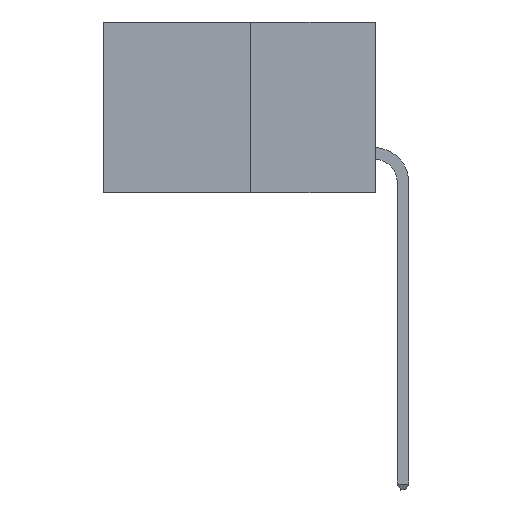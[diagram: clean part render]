
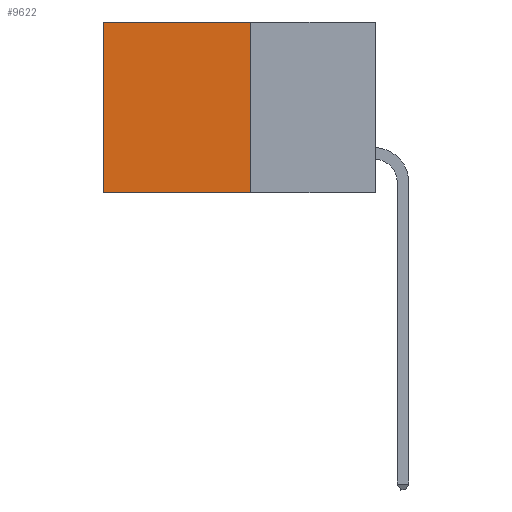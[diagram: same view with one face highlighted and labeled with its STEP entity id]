
A CAD part, left-side view. The second image highlights one B-rep face of the part: STEP entity #9622.
In plain terms, the highlighted planar face has unit normal (-1, 0, 0).
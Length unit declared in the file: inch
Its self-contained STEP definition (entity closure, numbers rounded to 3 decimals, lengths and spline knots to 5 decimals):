
#158 = DIRECTION ( 'NONE',  ( 0., 0., -1. ) ) ;
#978 = VERTEX_POINT ( 'NONE', #2963 ) ;
#1061 = CARTESIAN_POINT ( 'NONE',  ( 0.277, 0.27, -0.37 ) ) ;
#1401 = DIRECTION ( 'NONE',  ( 0., 1., 0. ) ) ;
#1878 = LINE ( 'NONE', #3910, #11128 ) ;
#1903 = CARTESIAN_POINT ( 'NONE',  ( 0.277, 0.59, 0. ) ) ;
#2042 = EDGE_CURVE ( 'NONE', #10965, #3764, #6798, .T. ) ;
#2249 = LINE ( 'NONE', #8948, #11425 ) ;
#2716 = LINE ( 'NONE', #9344, #7284 ) ;
#2913 = FACE_OUTER_BOUND ( 'NONE', #7314, .T. ) ;
#2963 = CARTESIAN_POINT ( 'NONE',  ( 0.277, 0.27, 0. ) ) ;
#3764 = VERTEX_POINT ( 'NONE', #4162 ) ;
#3910 = CARTESIAN_POINT ( 'NONE',  ( 0.277, 0.27, 0. ) ) ;
#3942 = AXIS2_PLACEMENT_3D ( 'NONE', #9145, #4697, #10850 ) ;
#4162 = CARTESIAN_POINT ( 'NONE',  ( 0.277, 0.59, -0.37 ) ) ;
#4377 = VECTOR ( 'NONE', #1401, 39.37008 ) ;
#4656 = PLANE ( 'NONE',  #3942 ) ;
#4697 = DIRECTION ( 'NONE',  ( 1., 0., 0. ) ) ;
#4829 = DIRECTION ( 'NONE',  ( 0., 1., 0. ) ) ;
#5393 = VERTEX_POINT ( 'NONE', #1903 ) ;
#6234 = EDGE_CURVE ( 'NONE', #978, #10965, #2249, .T. ) ;
#6798 = LINE ( 'NONE', #10276, #4377 ) ;
#7284 = VECTOR ( 'NONE', #158, 39.37008 ) ;
#7314 = EDGE_LOOP ( 'NONE', ( #7515, #7548, #7600, #7674 ) ) ;
#7515 = ORIENTED_EDGE ( 'NONE', *, *, #11017, .T. ) ;
#7548 = ORIENTED_EDGE ( 'NONE', *, *, #2042, .F. ) ;
#7600 = ORIENTED_EDGE ( 'NONE', *, *, #6234, .F. ) ;
#7674 = ORIENTED_EDGE ( 'NONE', *, *, #8668, .T. ) ;
#8668 = EDGE_CURVE ( 'NONE', #978, #5393, #1878, .T. ) ;
#8841 = DIRECTION ( 'NONE',  ( 0., 0., -1. ) ) ;
#8948 = CARTESIAN_POINT ( 'NONE',  ( 0.277, 0.27, -0.37 ) ) ;
#9145 = CARTESIAN_POINT ( 'NONE',  ( 0.277, 0.27, -0.37 ) ) ;
#9344 = CARTESIAN_POINT ( 'NONE',  ( 0.277, 0.59, -0.37 ) ) ;
#9622 = ADVANCED_FACE ( 'NONE', ( #2913 ), #4656, .F. ) ;
#10276 = CARTESIAN_POINT ( 'NONE',  ( 0.277, 0.27, -0.37 ) ) ;
#10850 = DIRECTION ( 'NONE',  ( 0., 0., -1. ) ) ;
#10965 = VERTEX_POINT ( 'NONE', #1061 ) ;
#11017 = EDGE_CURVE ( 'NONE', #5393, #3764, #2716, .T. ) ;
#11128 = VECTOR ( 'NONE', #4829, 39.37008 ) ;
#11425 = VECTOR ( 'NONE', #8841, 39.37008 ) ;
